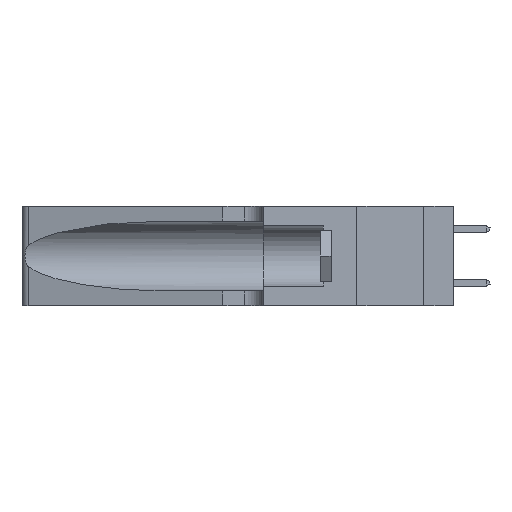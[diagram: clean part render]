
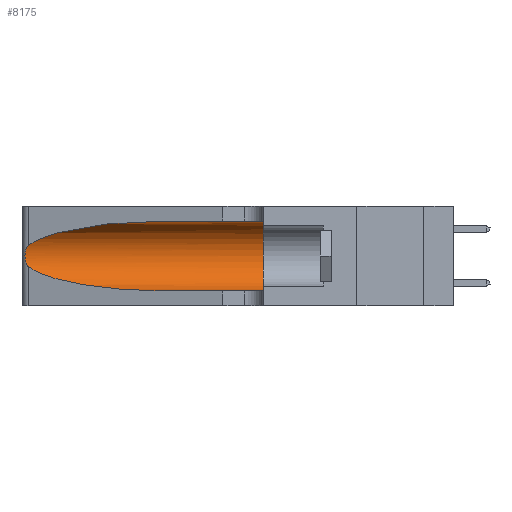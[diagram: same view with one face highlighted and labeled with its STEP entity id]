
A CAD part, left-side view. The second image highlights one B-rep face of the part: STEP entity #8175.
In plain terms, the highlighted cylindrical face has radius 3.308 mm (diameter 6.617 mm), a partial arc.
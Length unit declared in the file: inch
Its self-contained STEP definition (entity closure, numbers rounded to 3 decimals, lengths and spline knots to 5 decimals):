
#490 = CARTESIAN_POINT ( 'NONE',  ( 0.25639, 1.23186, 0.15144 ) ) ;
#638 = CARTESIAN_POINT ( 'NONE',  ( 0.18966, 0.96281, 0.31525 ) ) ;
#727 = ORIENTED_EDGE ( 'NONE', *, *, #24486, .T. ) ;
#1273 = EDGE_CURVE ( 'NONE', #18169, #12804, #11671, .T. ) ;
#1808 = EDGE_LOOP ( 'NONE', ( #13672, #727, #3429, #23074, #7294, #12970 ) ) ;
#1920 =( BOUNDED_CURVE ( )  B_SPLINE_CURVE ( 3, ( #7635, #23463, #2304, #9613 ),
 .UNSPECIFIED., .F., .T. ) 
 B_SPLINE_CURVE_WITH_KNOTS ( ( 4, 4 ),
 ( 3.44316, 4.71239 ),
 .UNSPECIFIED. ) 
 CURVE ( )  GEOMETRIC_REPRESENTATION_ITEM ( )  RATIONAL_B_SPLINE_CURVE ( ( 1., 0.87, 0.87, 1. ) ) 
 REPRESENTATION_ITEM ( '' )  );
#2064 = VERTEX_POINT ( 'NONE', #23716 ) ;
#2304 = CARTESIAN_POINT ( 'NONE',  ( 0.18966, 0.96281, 0.05475 ) ) ;
#3154 = DIRECTION ( 'NONE',  ( 0., 0., -1. ) ) ;
#3325 = CARTESIAN_POINT ( 'NONE',  ( 0.1305, 0.35, 0.31525 ) ) ;
#3429 = ORIENTED_EDGE ( 'NONE', *, *, #19221, .T. ) ;
#4096 = CARTESIAN_POINT ( 'NONE',  ( 0.1305, 0.35, 0.185 ) ) ;
#4128 = CARTESIAN_POINT ( 'NONE',  ( 0.25555, 1.22994, 0.2215 ) ) ;
#4192 = DIRECTION ( 'NONE',  ( 0., -1., 0. ) ) ;
#4298 = CARTESIAN_POINT ( 'NONE',  ( 0.25555, 1.22993, 0.14849 ) ) ;
#4957 = CARTESIAN_POINT ( 'NONE',  ( 0.25487, 1.22718, 0.22369 ) ) ;
#5609 = VERTEX_POINT ( 'NONE', #20223 ) ;
#6419 = CARTESIAN_POINT ( 'NONE',  ( 0.25854, 1.2359, 0.20912 ) ) ;
#6499 = CARTESIAN_POINT ( 'NONE',  ( 0.1305, 0.72297, 0.31525 ) ) ;
#6500 = CARTESIAN_POINT ( 'NONE',  ( 0.25487, 1.22718, 0.14631 ) ) ;
#6771 = AXIS2_PLACEMENT_3D ( 'NONE', #14687, #16703, #3154 ) ;
#7294 = ORIENTED_EDGE ( 'NONE', *, *, #18599, .F. ) ;
#7635 = CARTESIAN_POINT ( 'NONE',  ( 0.25487, 1.22718, 0.14631 ) ) ;
#8175 = ADVANCED_FACE ( 'NONE', ( #18848 ), #23022, .F. ) ;
#8435 = CARTESIAN_POINT ( 'NONE',  ( 0.2373, 1.15595, 0.28018 ) ) ;
#9613 = CARTESIAN_POINT ( 'NONE',  ( 0.1305, 0.72297, 0.05475 ) ) ;
#10071 = CARTESIAN_POINT ( 'NONE',  ( 0.26075, 1.23896, 0.19203 ) ) ;
#10117 = EDGE_CURVE ( 'NONE', #2064, #24692, #19613, .T. ) ;
#10309 = CARTESIAN_POINT ( 'NONE',  ( 0.25856, 1.23593, 0.16098 ) ) ;
#10398 = CARTESIAN_POINT ( 'NONE',  ( 0.26017, 1.23833, 0.17102 ) ) ;
#10461 = CARTESIAN_POINT ( 'NONE',  ( 0.25487, 1.22718, 0.22369 ) ) ;
#11671 =( BOUNDED_CURVE ( )  B_SPLINE_CURVE ( 3, ( #20269, #638, #8435, #10461 ),
 .UNSPECIFIED., .F., .T. ) 
 B_SPLINE_CURVE_WITH_KNOTS ( ( 4, 4 ),
 ( 1.5708, 2.84003 ),
 .UNSPECIFIED. ) 
 CURVE ( )  GEOMETRIC_REPRESENTATION_ITEM ( )  RATIONAL_B_SPLINE_CURVE ( ( 1., 0.87, 0.87, 1. ) ) 
 REPRESENTATION_ITEM ( '' )  );
#12053 = CARTESIAN_POINT ( 'NONE',  ( 0.26018, 1.23835, 0.19895 ) ) ;
#12522 = DIRECTION ( 'NONE',  ( 0., -1., 0. ) ) ;
#12737 = CARTESIAN_POINT ( 'NONE',  ( 0.1305, 0.35, 0.05475 ) ) ;
#12804 = VERTEX_POINT ( 'NONE', #4957 ) ;
#12964 = CIRCLE ( 'NONE', #16153, 0.13025 ) ;
#12970 = ORIENTED_EDGE ( 'NONE', *, *, #16770, .F. ) ;
#13498 = CARTESIAN_POINT ( 'NONE',  ( 0.25487, 1.22718, 0.22369 ) ) ;
#13617 = VECTOR ( 'NONE', #4192, 39.37008 ) ;
#13672 = ORIENTED_EDGE ( 'NONE', *, *, #1273, .T. ) ;
#14254 = B_SPLINE_CURVE_WITH_KNOTS ( 'NONE', 3,
 ( #13498, #4128, #15370, #19707, #6419, #12053, #10071, #21768, #10398, #10309, #23676, #490, #4298, #6500 ),
 .UNSPECIFIED., .F., .F.,
 ( 4, 2, 2, 2, 2, 2, 4 ),
 ( 0., 0.00027, 0.00053, 0.00107, 0.0016, 0.00187, 0.00214 ),
 .UNSPECIFIED. ) ;
#14504 = LINE ( 'NONE', #22049, #17206 ) ;
#14687 = CARTESIAN_POINT ( 'NONE',  ( 0.1305, 1.61858, 0.185 ) ) ;
#15370 = CARTESIAN_POINT ( 'NONE',  ( 0.25639, 1.23184, 0.21858 ) ) ;
#15739 = CARTESIAN_POINT ( 'NONE',  ( 0.1305, 1.61858, 0.05475 ) ) ;
#16153 = AXIS2_PLACEMENT_3D ( 'NONE', #4096, #19259, #23401 ) ;
#16703 = DIRECTION ( 'NONE',  ( 0., -1., 0. ) ) ;
#16770 = EDGE_CURVE ( 'NONE', #18169, #19646, #14504, .T. ) ;
#17206 = VECTOR ( 'NONE', #12522, 39.37008 ) ;
#18169 = VERTEX_POINT ( 'NONE', #6499 ) ;
#18599 = EDGE_CURVE ( 'NONE', #19646, #24692, #12964, .T. ) ;
#18848 = FACE_OUTER_BOUND ( 'NONE', #1808, .T. ) ;
#19221 = EDGE_CURVE ( 'NONE', #5609, #2064, #1920, .T. ) ;
#19259 = DIRECTION ( 'NONE',  ( 0., 1., 0. ) ) ;
#19613 = LINE ( 'NONE', #15739, #13617 ) ;
#19646 = VERTEX_POINT ( 'NONE', #3325 ) ;
#19707 = CARTESIAN_POINT ( 'NONE',  ( 0.25787, 1.23484, 0.2124 ) ) ;
#20223 = CARTESIAN_POINT ( 'NONE',  ( 0.25487, 1.22718, 0.14631 ) ) ;
#20269 = CARTESIAN_POINT ( 'NONE',  ( 0.1305, 0.72297, 0.31525 ) ) ;
#21768 = CARTESIAN_POINT ( 'NONE',  ( 0.26075, 1.23896, 0.178 ) ) ;
#22049 = CARTESIAN_POINT ( 'NONE',  ( 0.1305, 1.61858, 0.31525 ) ) ;
#23022 = CYLINDRICAL_SURFACE ( 'NONE', #6771, 0.13025 ) ;
#23074 = ORIENTED_EDGE ( 'NONE', *, *, #10117, .T. ) ;
#23401 = DIRECTION ( 'NONE',  ( 0., 0., 1. ) ) ;
#23463 = CARTESIAN_POINT ( 'NONE',  ( 0.2373, 1.15595, 0.08982 ) ) ;
#23676 = CARTESIAN_POINT ( 'NONE',  ( 0.25789, 1.23486, 0.15765 ) ) ;
#23716 = CARTESIAN_POINT ( 'NONE',  ( 0.1305, 0.72297, 0.05475 ) ) ;
#24486 = EDGE_CURVE ( 'NONE', #12804, #5609, #14254, .T. ) ;
#24692 = VERTEX_POINT ( 'NONE', #12737 ) ;
